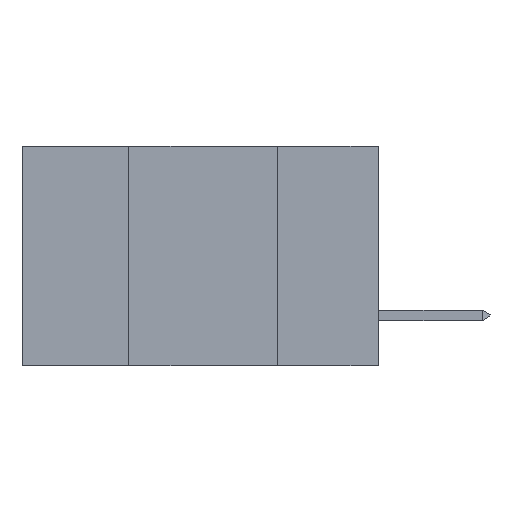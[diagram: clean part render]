
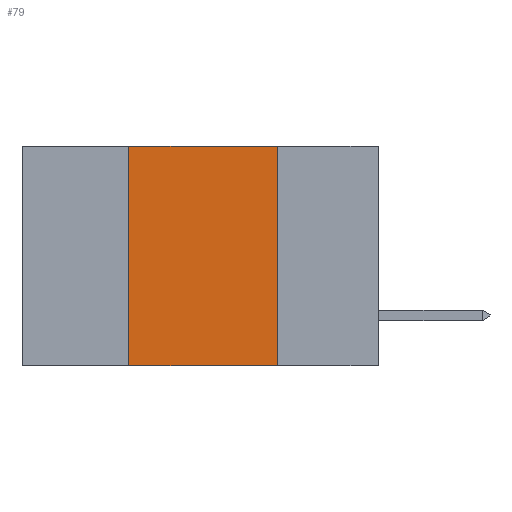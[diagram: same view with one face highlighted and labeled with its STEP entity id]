
A CAD part, left-side view. The second image highlights one B-rep face of the part: STEP entity #79.
In plain terms, the highlighted planar face has unit normal (-1, 0, 0).
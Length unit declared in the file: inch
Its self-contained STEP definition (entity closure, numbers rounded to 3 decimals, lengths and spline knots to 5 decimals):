
#79 = ADVANCED_FACE ( 'NONE', ( #9937 ), #5771, .F. ) ;
#115 = CARTESIAN_POINT ( 'NONE',  ( 0., 0.42, -0.37 ) ) ;
#280 = ORIENTED_EDGE ( 'NONE', *, *, #8344, .F. ) ;
#825 = CARTESIAN_POINT ( 'NONE',  ( 0., 0.17, -0.37 ) ) ;
#875 = EDGE_CURVE ( 'NONE', #6145, #7226, #1483, .T. ) ;
#1483 = LINE ( 'NONE', #10176, #3670 ) ;
#1856 = ORIENTED_EDGE ( 'NONE', *, *, #875, .T. ) ;
#2229 = DIRECTION ( 'NONE',  ( 0., 0., 1. ) ) ;
#2384 = DIRECTION ( 'NONE',  ( 0., -1., 0. ) ) ;
#2443 = ORIENTED_EDGE ( 'NONE', *, *, #10859, .F. ) ;
#3190 = VERTEX_POINT ( 'NONE', #8309 ) ;
#3449 = CARTESIAN_POINT ( 'NONE',  ( 0., 0.17, 0. ) ) ;
#3657 = VECTOR ( 'NONE', #2229, 39.37008 ) ;
#3670 = VECTOR ( 'NONE', #2384, 39.37008 ) ;
#4797 = LINE ( 'NONE', #6391, #3657 ) ;
#4848 = DIRECTION ( 'NONE',  ( 0., 0., -1. ) ) ;
#4913 = DIRECTION ( 'NONE',  ( 0., -1., 0. ) ) ;
#4933 = DIRECTION ( 'NONE',  ( 1., 0., 0. ) ) ;
#5519 = CARTESIAN_POINT ( 'NONE',  ( 0., 0.17, -0.37 ) ) ;
#5771 = PLANE ( 'NONE',  #9632 ) ;
#6145 = VERTEX_POINT ( 'NONE', #115 ) ;
#6391 = CARTESIAN_POINT ( 'NONE',  ( 0., 0.42, -0.37 ) ) ;
#7226 = VERTEX_POINT ( 'NONE', #825 ) ;
#7694 = VERTEX_POINT ( 'NONE', #3449 ) ;
#8037 = VECTOR ( 'NONE', #4913, 39.37008 ) ;
#8137 = LINE ( 'NONE', #9054, #8037 ) ;
#8309 = CARTESIAN_POINT ( 'NONE',  ( 0., 0.42, 0. ) ) ;
#8344 = EDGE_CURVE ( 'NONE', #6145, #3190, #4797, .T. ) ;
#8419 = VECTOR ( 'NONE', #4848, 39.37008 ) ;
#8620 = ORIENTED_EDGE ( 'NONE', *, *, #11165, .F. ) ;
#9054 = CARTESIAN_POINT ( 'NONE',  ( 0., 0.6, 0. ) ) ;
#9238 = CARTESIAN_POINT ( 'NONE',  ( 0., 0.6, 0. ) ) ;
#9414 = EDGE_LOOP ( 'NONE', ( #8620, #2443, #280, #1856 ) ) ;
#9632 = AXIS2_PLACEMENT_3D ( 'NONE', #9238, #4933, #10156 ) ;
#9937 = FACE_OUTER_BOUND ( 'NONE', #9414, .T. ) ;
#10156 = DIRECTION ( 'NONE',  ( 0., 0., -1. ) ) ;
#10176 = CARTESIAN_POINT ( 'NONE',  ( 0., 0.6, -0.37 ) ) ;
#10859 = EDGE_CURVE ( 'NONE', #3190, #7694, #8137, .T. ) ;
#10860 = LINE ( 'NONE', #5519, #8419 ) ;
#11165 = EDGE_CURVE ( 'NONE', #7694, #7226, #10860, .T. ) ;
